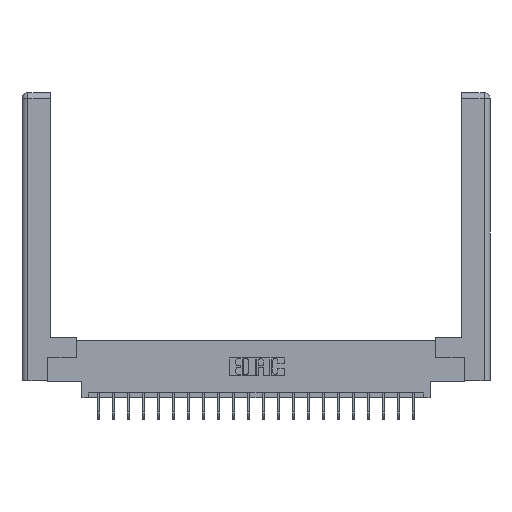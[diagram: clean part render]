
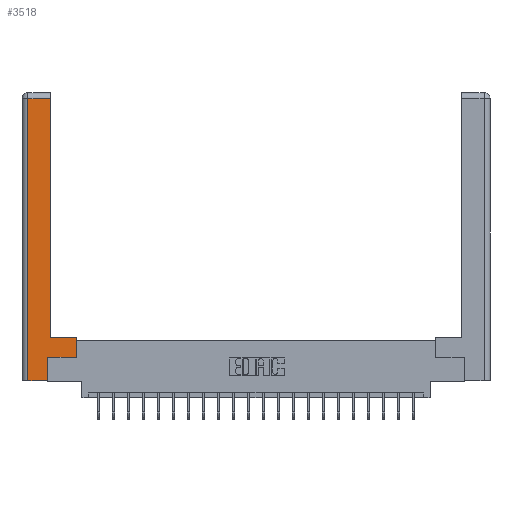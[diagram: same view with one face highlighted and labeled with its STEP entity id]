
A CAD part, top view. The second image highlights one B-rep face of the part: STEP entity #3518.
In plain terms, the highlighted planar face has unit normal (0, 0, 1).
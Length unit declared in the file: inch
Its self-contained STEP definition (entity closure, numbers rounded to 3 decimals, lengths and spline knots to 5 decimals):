
#611 = VECTOR ( 'NONE', #10266, 39.37008 ) ;
#1375 = CARTESIAN_POINT ( 'NONE',  ( 0.265, 0., 0. ) ) ;
#1472 = DIRECTION ( 'NONE',  ( -1., 0., 0. ) ) ;
#1970 = VERTEX_POINT ( 'NONE', #20638 ) ;
#2202 = VECTOR ( 'NONE', #19720, 39.37008 ) ;
#2511 = CARTESIAN_POINT ( 'NONE',  ( 0.0615, 0., 0. ) ) ;
#2765 = DIRECTION ( 'NONE',  ( 0., 1., 0. ) ) ;
#3369 = LINE ( 'NONE', #20204, #22685 ) ;
#3518 = ADVANCED_FACE ( 'NONE', ( #8588 ), #12668, .F. ) ;
#4152 = CARTESIAN_POINT ( 'NONE',  ( 0.0615, 2.94, 0. ) ) ;
#4238 = DIRECTION ( 'NONE',  ( -1., 0., 0. ) ) ;
#4580 = EDGE_LOOP ( 'NONE', ( #19683, #4966, #5092, #18059, #22842, #11307, #5446, #21167 ) ) ;
#4680 = LINE ( 'NONE', #14802, #22468 ) ;
#4748 = CARTESIAN_POINT ( 'NONE',  ( 0.565, 0.45, 0. ) ) ;
#4828 = LINE ( 'NONE', #7737, #20877 ) ;
#4966 = ORIENTED_EDGE ( 'NONE', *, *, #19800, .T. ) ;
#4969 = LINE ( 'NONE', #9145, #9915 ) ;
#5092 = ORIENTED_EDGE ( 'NONE', *, *, #8399, .T. ) ;
#5224 = DIRECTION ( 'NONE',  ( 0., -1., 0. ) ) ;
#5446 = ORIENTED_EDGE ( 'NONE', *, *, #16046, .T. ) ;
#5487 = VERTEX_POINT ( 'NONE', #2511 ) ;
#5711 = DIRECTION ( 'NONE',  ( 1., 0., 0. ) ) ;
#6242 = VECTOR ( 'NONE', #4238, 39.37008 ) ;
#6353 = EDGE_CURVE ( 'NONE', #19154, #15516, #4680, .T. ) ;
#7189 = LINE ( 'NONE', #20027, #2202 ) ;
#7297 = DIRECTION ( 'NONE',  ( -1., 0., 0. ) ) ;
#7737 = CARTESIAN_POINT ( 'NONE',  ( 0.265, 0., 0. ) ) ;
#8049 = CARTESIAN_POINT ( 'NONE',  ( 0.295, 2.94, 0. ) ) ;
#8205 = LINE ( 'NONE', #19472, #611 ) ;
#8399 = EDGE_CURVE ( 'NONE', #17549, #5487, #3369, .T. ) ;
#8450 = CARTESIAN_POINT ( 'NONE',  ( 0.565, 0.45, 0. ) ) ;
#8588 = FACE_OUTER_BOUND ( 'NONE', #4580, .T. ) ;
#9145 = CARTESIAN_POINT ( 'NONE',  ( 0.265, 0.245, 0. ) ) ;
#9427 = AXIS2_PLACEMENT_3D ( 'NONE', #22227, #22313, #1472 ) ;
#9915 = VECTOR ( 'NONE', #11104, 39.37008 ) ;
#9921 = LINE ( 'NONE', #4748, #20436 ) ;
#10266 = DIRECTION ( 'NONE',  ( 0., 1., 0. ) ) ;
#10503 = VERTEX_POINT ( 'NONE', #1375 ) ;
#11073 = CARTESIAN_POINT ( 'NONE',  ( 0.565, 0.245, 0. ) ) ;
#11079 = EDGE_CURVE ( 'NONE', #15516, #21652, #8205, .T. ) ;
#11104 = DIRECTION ( 'NONE',  ( 0., 1., 0. ) ) ;
#11307 = ORIENTED_EDGE ( 'NONE', *, *, #17903, .T. ) ;
#11771 = EDGE_CURVE ( 'NONE', #10503, #1970, #4969, .T. ) ;
#12668 = PLANE ( 'NONE',  #9427 ) ;
#14802 = CARTESIAN_POINT ( 'NONE',  ( 0.295, 0.45, 0. ) ) ;
#15516 = VERTEX_POINT ( 'NONE', #23553 ) ;
#16046 = EDGE_CURVE ( 'NONE', #16320, #19154, #9921, .T. ) ;
#16320 = VERTEX_POINT ( 'NONE', #11073 ) ;
#16723 = LINE ( 'NONE', #4152, #6242 ) ;
#17549 = VERTEX_POINT ( 'NONE', #18890 ) ;
#17903 = EDGE_CURVE ( 'NONE', #1970, #16320, #7189, .T. ) ;
#18059 = ORIENTED_EDGE ( 'NONE', *, *, #20889, .T. ) ;
#18890 = CARTESIAN_POINT ( 'NONE',  ( 0.0615, 2.94, 0. ) ) ;
#19154 = VERTEX_POINT ( 'NONE', #8450 ) ;
#19472 = CARTESIAN_POINT ( 'NONE',  ( 0.295, 3., 0. ) ) ;
#19683 = ORIENTED_EDGE ( 'NONE', *, *, #11079, .T. ) ;
#19720 = DIRECTION ( 'NONE',  ( 1., 0., 0. ) ) ;
#19800 = EDGE_CURVE ( 'NONE', #21652, #17549, #16723, .T. ) ;
#20027 = CARTESIAN_POINT ( 'NONE',  ( 0.565, 0.245, 0. ) ) ;
#20204 = CARTESIAN_POINT ( 'NONE',  ( 0.0615, 0., 0. ) ) ;
#20436 = VECTOR ( 'NONE', #2765, 39.37008 ) ;
#20638 = CARTESIAN_POINT ( 'NONE',  ( 0.265, 0.245, 0. ) ) ;
#20877 = VECTOR ( 'NONE', #5711, 39.37008 ) ;
#20889 = EDGE_CURVE ( 'NONE', #5487, #10503, #4828, .T. ) ;
#21167 = ORIENTED_EDGE ( 'NONE', *, *, #6353, .T. ) ;
#21652 = VERTEX_POINT ( 'NONE', #8049 ) ;
#22227 = CARTESIAN_POINT ( 'NONE',  ( 0., 0., 0. ) ) ;
#22313 = DIRECTION ( 'NONE',  ( 0., 0., -1. ) ) ;
#22468 = VECTOR ( 'NONE', #7297, 39.37008 ) ;
#22685 = VECTOR ( 'NONE', #5224, 39.37008 ) ;
#22842 = ORIENTED_EDGE ( 'NONE', *, *, #11771, .T. ) ;
#23553 = CARTESIAN_POINT ( 'NONE',  ( 0.295, 0.45, 0. ) ) ;
